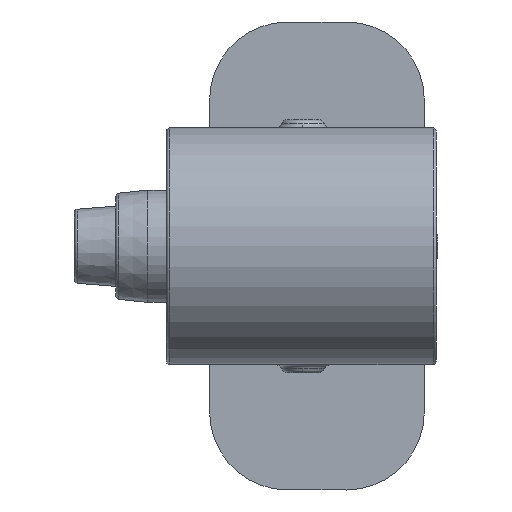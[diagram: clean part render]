
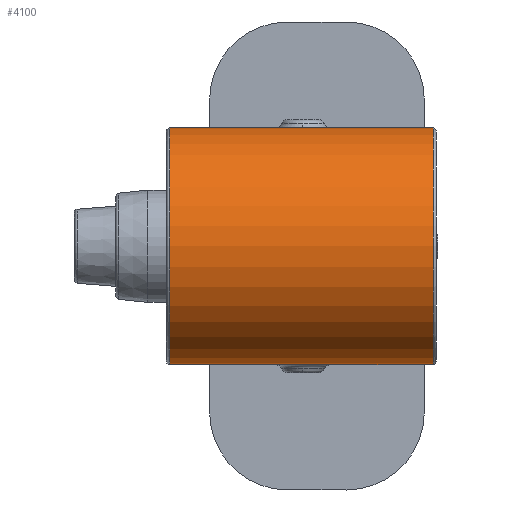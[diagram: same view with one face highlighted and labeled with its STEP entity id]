
A CAD part, left-side view. The second image highlights one B-rep face of the part: STEP entity #4100.
In plain terms, the highlighted cylindrical face has radius 3.7 mm (diameter 7.4 mm), a partial arc.
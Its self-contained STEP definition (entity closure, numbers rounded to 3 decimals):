
#77 = AXIS2_PLACEMENT_3D ( 'NONE', #5358, #2301, #4929 ) ;
#97 = ORIENTED_EDGE ( 'NONE', *, *, #2748, .F. ) ;
#504 = CIRCLE ( 'NONE', #77, 3.7 ) ;
#797 = VERTEX_POINT ( 'NONE', #6165 ) ;
#887 = CARTESIAN_POINT ( 'NONE',  ( -7.6, 8.32, -3.7 ) ) ;
#1336 = DIRECTION ( 'NONE',  ( 0., -1., 0. ) ) ;
#1750 = CARTESIAN_POINT ( 'NONE',  ( -7.6, 0.1, 3.7 ) ) ;
#2098 = EDGE_CURVE ( 'NONE', #3229, #4246, #504, .T. ) ;
#2301 = DIRECTION ( 'NONE',  ( 0., 1., 0. ) ) ;
#2550 = VECTOR ( 'NONE', #2973, 1000. ) ;
#2585 = EDGE_CURVE ( 'NONE', #3583, #3229, #5986, .T. ) ;
#2748 = EDGE_CURVE ( 'NONE', #797, #4246, #5442, .T. ) ;
#2795 = AXIS2_PLACEMENT_3D ( 'NONE', #4783, #5273, #6269 ) ;
#2951 = AXIS2_PLACEMENT_3D ( 'NONE', #5875, #1336, #3355 ) ;
#2973 = DIRECTION ( 'NONE',  ( 0., -1., 0. ) ) ;
#3229 = VERTEX_POINT ( 'NONE', #3477 ) ;
#3355 = DIRECTION ( 'NONE',  ( 0., 0., -1. ) ) ;
#3477 = CARTESIAN_POINT ( 'NONE',  ( -7.6, 0.1, -3.7 ) ) ;
#3583 = VERTEX_POINT ( 'NONE', #887 ) ;
#3715 = VECTOR ( 'NONE', #6499, 1000. ) ;
#3866 = FACE_OUTER_BOUND ( 'NONE', #4071, .T. ) ;
#3896 = EDGE_CURVE ( 'NONE', #797, #3583, #4921, .T. ) ;
#4071 = EDGE_LOOP ( 'NONE', ( #4133, #5636, #97, #6029 ) ) ;
#4100 = ADVANCED_FACE ( 'NONE', ( #3866 ), #4884, .T. ) ;
#4133 = ORIENTED_EDGE ( 'NONE', *, *, #2585, .T. ) ;
#4246 = VERTEX_POINT ( 'NONE', #1750 ) ;
#4415 = CARTESIAN_POINT ( 'NONE',  ( -7.6, 8.42, -3.7 ) ) ;
#4783 = CARTESIAN_POINT ( 'NONE',  ( -7.6, 8.32, 0. ) ) ;
#4884 = CYLINDRICAL_SURFACE ( 'NONE', #2951, 3.7 ) ;
#4921 = CIRCLE ( 'NONE', #2795, 3.7 ) ;
#4929 = DIRECTION ( 'NONE',  ( 0., 0., 1. ) ) ;
#5273 = DIRECTION ( 'NONE',  ( 0., -1., 0. ) ) ;
#5358 = CARTESIAN_POINT ( 'NONE',  ( -7.6, 0.1, 0. ) ) ;
#5442 = LINE ( 'NONE', #5994, #3715 ) ;
#5636 = ORIENTED_EDGE ( 'NONE', *, *, #2098, .T. ) ;
#5875 = CARTESIAN_POINT ( 'NONE',  ( -7.6, 8.42, 0. ) ) ;
#5986 = LINE ( 'NONE', #4415, #2550 ) ;
#5994 = CARTESIAN_POINT ( 'NONE',  ( -7.6, 8.42, 3.7 ) ) ;
#6029 = ORIENTED_EDGE ( 'NONE', *, *, #3896, .T. ) ;
#6165 = CARTESIAN_POINT ( 'NONE',  ( -7.6, 8.32, 3.7 ) ) ;
#6269 = DIRECTION ( 'NONE',  ( 0., 0., 1. ) ) ;
#6499 = DIRECTION ( 'NONE',  ( 0., -1., 0. ) ) ;
